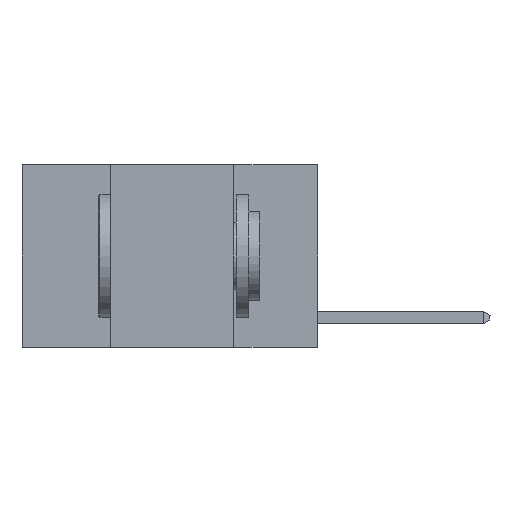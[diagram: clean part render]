
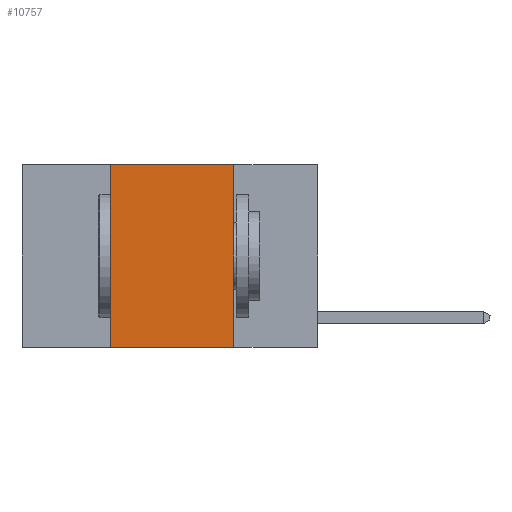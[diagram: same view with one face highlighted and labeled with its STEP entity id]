
A CAD part, left-side view. The second image highlights one B-rep face of the part: STEP entity #10757.
In plain terms, the highlighted planar face has unit normal (-1, 0, 0).
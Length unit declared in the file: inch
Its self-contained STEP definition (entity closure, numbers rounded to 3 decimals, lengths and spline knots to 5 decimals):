
#628 = VERTEX_POINT ( 'NONE', #6507 ) ;
#1078 = VERTEX_POINT ( 'NONE', #3864 ) ;
#1192 = VECTOR ( 'NONE', #12018, 39.37008 ) ;
#1622 = DIRECTION ( 'NONE',  ( 0., 0., -1. ) ) ;
#1690 = EDGE_CURVE ( 'NONE', #13579, #12051, #12126, .T. ) ;
#1993 = EDGE_CURVE ( 'NONE', #13579, #628, #13916, .T. ) ;
#3137 = DIRECTION ( 'NONE',  ( 0., 0., -1. ) ) ;
#3824 = DIRECTION ( 'NONE',  ( 1., 0., 0. ) ) ;
#3864 = CARTESIAN_POINT ( 'NONE',  ( 0., 0.17, 0. ) ) ;
#3894 = ORIENTED_EDGE ( 'NONE', *, *, #1690, .F. ) ;
#4164 = CARTESIAN_POINT ( 'NONE',  ( 0., 0.6, -0.37 ) ) ;
#4174 = ORIENTED_EDGE ( 'NONE', *, *, #7671, .F. ) ;
#4798 = EDGE_CURVE ( 'NONE', #12051, #1078, #6350, .T. ) ;
#5491 = DIRECTION ( 'NONE',  ( 0., -1., 0. ) ) ;
#5602 = ORIENTED_EDGE ( 'NONE', *, *, #4798, .F. ) ;
#5803 = CARTESIAN_POINT ( 'NONE',  ( 0., 0.42, -0.37 ) ) ;
#6120 = AXIS2_PLACEMENT_3D ( 'NONE', #7012, #3824, #1622 ) ;
#6350 = LINE ( 'NONE', #10849, #7400 ) ;
#6507 = CARTESIAN_POINT ( 'NONE',  ( 0., 0.17, -0.37 ) ) ;
#6668 = CARTESIAN_POINT ( 'NONE',  ( 0., 0.42, 0. ) ) ;
#6939 = FACE_OUTER_BOUND ( 'NONE', #9633, .T. ) ;
#7012 = CARTESIAN_POINT ( 'NONE',  ( 0., 0.6, 0. ) ) ;
#7027 = CARTESIAN_POINT ( 'NONE',  ( 0., 0.42, 0. ) ) ;
#7400 = VECTOR ( 'NONE', #5491, 39.37008 ) ;
#7671 = EDGE_CURVE ( 'NONE', #1078, #628, #8385, .T. ) ;
#7997 = PLANE ( 'NONE',  #6120 ) ;
#8385 = LINE ( 'NONE', #10620, #9934 ) ;
#9633 = EDGE_LOOP ( 'NONE', ( #4174, #5602, #3894, #10981 ) ) ;
#9934 = VECTOR ( 'NONE', #3137, 39.37008 ) ;
#10491 = VECTOR ( 'NONE', #11907, 39.37008 ) ;
#10620 = CARTESIAN_POINT ( 'NONE',  ( 0., 0.17, 0. ) ) ;
#10757 = ADVANCED_FACE ( 'NONE', ( #6939 ), #7997, .F. ) ;
#10849 = CARTESIAN_POINT ( 'NONE',  ( 0., 0.6, 0. ) ) ;
#10981 = ORIENTED_EDGE ( 'NONE', *, *, #1993, .T. ) ;
#11907 = DIRECTION ( 'NONE',  ( 0., 0., 1. ) ) ;
#12018 = DIRECTION ( 'NONE',  ( 0., -1., 0. ) ) ;
#12051 = VERTEX_POINT ( 'NONE', #7027 ) ;
#12126 = LINE ( 'NONE', #6668, #10491 ) ;
#13579 = VERTEX_POINT ( 'NONE', #5803 ) ;
#13916 = LINE ( 'NONE', #4164, #1192 ) ;
